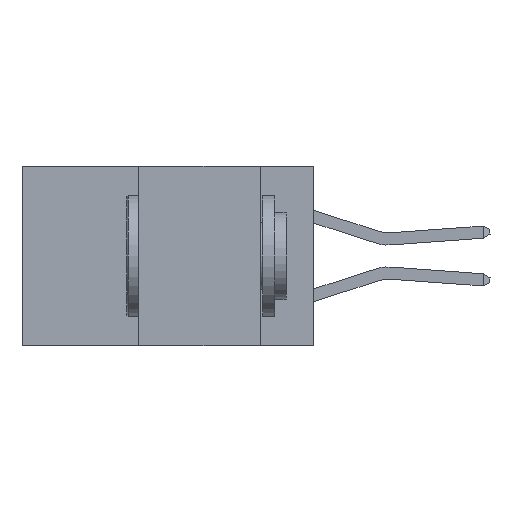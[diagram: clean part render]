
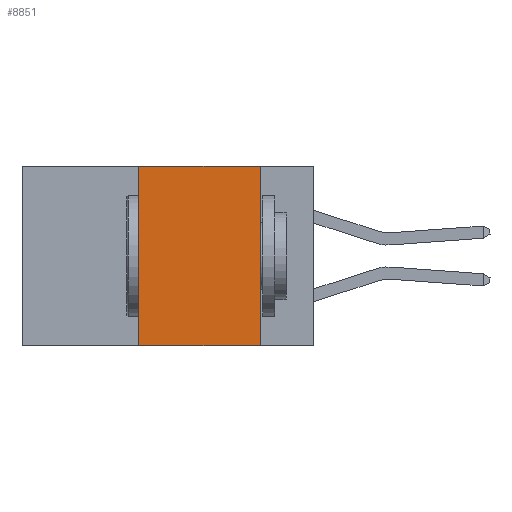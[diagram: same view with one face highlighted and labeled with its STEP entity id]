
A CAD part, left-side view. The second image highlights one B-rep face of the part: STEP entity #8851.
In plain terms, the highlighted planar face has unit normal (-1, 0, 0).
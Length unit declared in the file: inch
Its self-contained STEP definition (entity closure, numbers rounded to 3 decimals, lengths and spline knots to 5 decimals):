
#438 = VERTEX_POINT ( 'NONE', #22380 ) ;
#592 = LINE ( 'NONE', #8532, #13828 ) ;
#1042 = CARTESIAN_POINT ( 'NONE',  ( 0., 0.36, 0. ) ) ;
#2352 = DIRECTION ( 'NONE',  ( 0., 0., -1. ) ) ;
#3255 = CARTESIAN_POINT ( 'NONE',  ( 0., 0.11, 0. ) ) ;
#3682 = DIRECTION ( 'NONE',  ( 0., 0., -1. ) ) ;
#3705 = DIRECTION ( 'NONE',  ( 0., 0., 1. ) ) ;
#3789 = FACE_OUTER_BOUND ( 'NONE', #16414, .T. ) ;
#3918 = ORIENTED_EDGE ( 'NONE', *, *, #7309, .F. ) ;
#6802 = CARTESIAN_POINT ( 'NONE',  ( 0., 0.36, 0. ) ) ;
#7309 = EDGE_CURVE ( 'NONE', #32362, #438, #8855, .T. ) ;
#8005 = VERTEX_POINT ( 'NONE', #6802 ) ;
#8532 = CARTESIAN_POINT ( 'NONE',  ( 0., 0.6, -0.37 ) ) ;
#8851 = ADVANCED_FACE ( 'NONE', ( #3789 ), #12847, .F. ) ;
#8855 = LINE ( 'NONE', #24591, #14222 ) ;
#9441 = LINE ( 'NONE', #33207, #15640 ) ;
#9876 = DIRECTION ( 'NONE',  ( 0., -1., 0. ) ) ;
#10841 = CARTESIAN_POINT ( 'NONE',  ( 0., 0.36, -0.37 ) ) ;
#11195 = DIRECTION ( 'NONE',  ( 0., -1., 0. ) ) ;
#12811 = EDGE_CURVE ( 'NONE', #13842, #438, #592, .T. ) ;
#12847 = PLANE ( 'NONE',  #18883 ) ;
#13828 = VECTOR ( 'NONE', #11195, 39.37008 ) ;
#13842 = VERTEX_POINT ( 'NONE', #10841 ) ;
#14222 = VECTOR ( 'NONE', #3682, 39.37008 ) ;
#15009 = ORIENTED_EDGE ( 'NONE', *, *, #20314, .F. ) ;
#15506 = CARTESIAN_POINT ( 'NONE',  ( 0., 0.6, 0. ) ) ;
#15640 = VECTOR ( 'NONE', #9876, 39.37008 ) ;
#16414 = EDGE_LOOP ( 'NONE', ( #3918, #32327, #15009, #26307 ) ) ;
#18135 = DIRECTION ( 'NONE',  ( 1., 0., 0. ) ) ;
#18345 = LINE ( 'NONE', #1042, #24460 ) ;
#18883 = AXIS2_PLACEMENT_3D ( 'NONE', #15506, #18135, #2352 ) ;
#20314 = EDGE_CURVE ( 'NONE', #13842, #8005, #18345, .T. ) ;
#22380 = CARTESIAN_POINT ( 'NONE',  ( 0., 0.11, -0.37 ) ) ;
#24460 = VECTOR ( 'NONE', #3705, 39.37008 ) ;
#24591 = CARTESIAN_POINT ( 'NONE',  ( 0., 0.11, 0. ) ) ;
#26307 = ORIENTED_EDGE ( 'NONE', *, *, #12811, .T. ) ;
#32327 = ORIENTED_EDGE ( 'NONE', *, *, #33385, .F. ) ;
#32362 = VERTEX_POINT ( 'NONE', #3255 ) ;
#33207 = CARTESIAN_POINT ( 'NONE',  ( 0., 0.6, 0. ) ) ;
#33385 = EDGE_CURVE ( 'NONE', #8005, #32362, #9441, .T. ) ;
